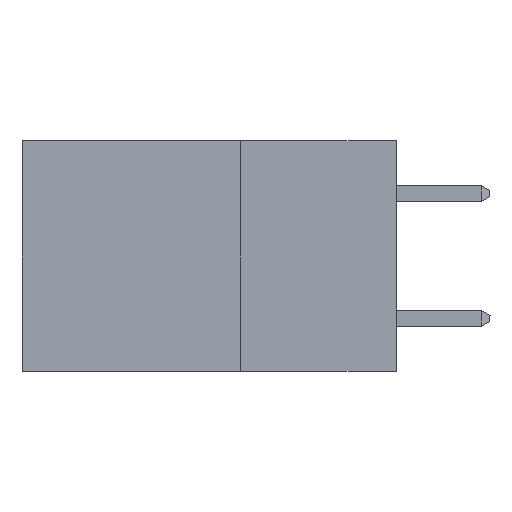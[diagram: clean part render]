
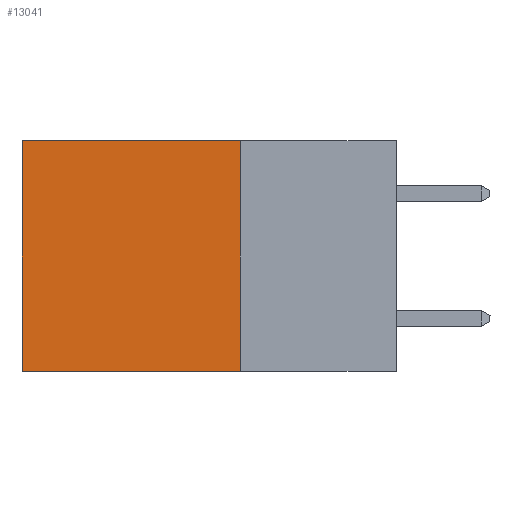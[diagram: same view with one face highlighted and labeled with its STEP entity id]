
A CAD part, left-side view. The second image highlights one B-rep face of the part: STEP entity #13041.
In plain terms, the highlighted planar face has unit normal (-1, 0, 0).
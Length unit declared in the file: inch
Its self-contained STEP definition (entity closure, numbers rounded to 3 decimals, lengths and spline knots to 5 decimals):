
#527 = VERTEX_POINT ( 'NONE', #9235 ) ;
#547 = EDGE_CURVE ( 'NONE', #8427, #8796, #2032, .T. ) ;
#646 = CARTESIAN_POINT ( 'NONE',  ( 0.2615, 0.6, -0.37 ) ) ;
#697 = ORIENTED_EDGE ( 'NONE', *, *, #2722, .T. ) ;
#1156 = VECTOR ( 'NONE', #3927, 39.37008 ) ;
#1487 = DIRECTION ( 'NONE',  ( 0., 0., -1. ) ) ;
#1647 = CARTESIAN_POINT ( 'NONE',  ( 0.2615, 0.6, -0.37 ) ) ;
#1855 = LINE ( 'NONE', #4345, #1156 ) ;
#2032 = LINE ( 'NONE', #8989, #13461 ) ;
#2298 = ORIENTED_EDGE ( 'NONE', *, *, #6848, .F. ) ;
#2677 = PLANE ( 'NONE',  #7744 ) ;
#2722 = EDGE_CURVE ( 'NONE', #5662, #527, #1855, .T. ) ;
#2724 = VECTOR ( 'NONE', #10405, 39.37008 ) ;
#3762 = DIRECTION ( 'NONE',  ( 1., 0., 0. ) ) ;
#3927 = DIRECTION ( 'NONE',  ( 0., 1., 0. ) ) ;
#4010 = VECTOR ( 'NONE', #1487, 39.37008 ) ;
#4062 = CARTESIAN_POINT ( 'NONE',  ( 0.2615, 0.25, 0. ) ) ;
#4280 = EDGE_CURVE ( 'NONE', #527, #8796, #4369, .T. ) ;
#4345 = CARTESIAN_POINT ( 'NONE',  ( 0.2615, 0.25, 0. ) ) ;
#4369 = LINE ( 'NONE', #1647, #4010 ) ;
#4668 = EDGE_LOOP ( 'NONE', ( #7083, #5590, #2298, #697 ) ) ;
#5590 = ORIENTED_EDGE ( 'NONE', *, *, #547, .F. ) ;
#5662 = VERTEX_POINT ( 'NONE', #4062 ) ;
#5720 = CARTESIAN_POINT ( 'NONE',  ( 0.2615, 0.25, -0.37 ) ) ;
#6848 = EDGE_CURVE ( 'NONE', #5662, #8427, #9066, .T. ) ;
#7083 = ORIENTED_EDGE ( 'NONE', *, *, #4280, .T. ) ;
#7744 = AXIS2_PLACEMENT_3D ( 'NONE', #10516, #3762, #11601 ) ;
#8427 = VERTEX_POINT ( 'NONE', #5720 ) ;
#8665 = DIRECTION ( 'NONE',  ( 0., 1., 0. ) ) ;
#8796 = VERTEX_POINT ( 'NONE', #646 ) ;
#8801 = FACE_OUTER_BOUND ( 'NONE', #4668, .T. ) ;
#8989 = CARTESIAN_POINT ( 'NONE',  ( 0.2615, 0.25, -0.37 ) ) ;
#9066 = LINE ( 'NONE', #10576, #2724 ) ;
#9235 = CARTESIAN_POINT ( 'NONE',  ( 0.2615, 0.6, 0. ) ) ;
#10405 = DIRECTION ( 'NONE',  ( 0., 0., -1. ) ) ;
#10516 = CARTESIAN_POINT ( 'NONE',  ( 0.2615, 0.25, -0.37 ) ) ;
#10576 = CARTESIAN_POINT ( 'NONE',  ( 0.2615, 0.25, -0.37 ) ) ;
#11601 = DIRECTION ( 'NONE',  ( 0., 0., -1. ) ) ;
#13041 = ADVANCED_FACE ( 'NONE', ( #8801 ), #2677, .F. ) ;
#13461 = VECTOR ( 'NONE', #8665, 39.37008 ) ;
